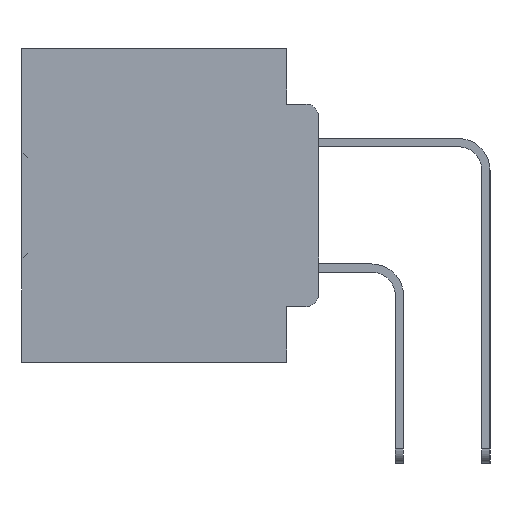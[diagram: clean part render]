
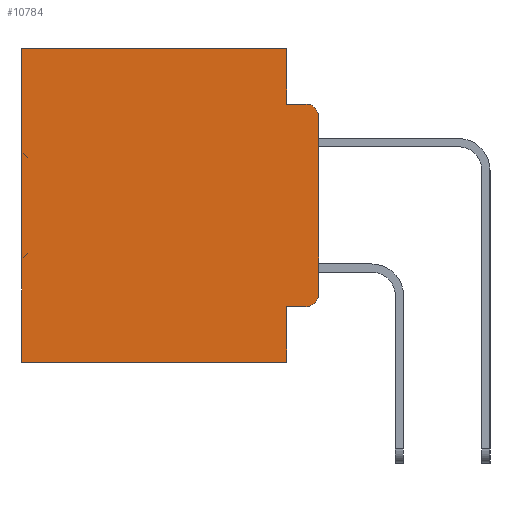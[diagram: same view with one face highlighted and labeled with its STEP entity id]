
A CAD part, left-side view. The second image highlights one B-rep face of the part: STEP entity #10784.
In plain terms, the highlighted planar face has unit normal (-1, 0, 0).
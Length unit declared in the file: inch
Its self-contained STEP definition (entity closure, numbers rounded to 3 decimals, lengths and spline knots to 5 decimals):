
#329 = DIRECTION ( 'NONE',  ( 0., 0., -1. ) ) ;
#488 = EDGE_LOOP ( 'NONE', ( #30533, #26511, #18700, #25436, #609, #20765, #15662, #32718, #24163, #22100 ) ) ;
#609 = ORIENTED_EDGE ( 'NONE', *, *, #13369, .T. ) ;
#620 = EDGE_CURVE ( 'NONE', #18896, #14443, #38742, .T. ) ;
#678 = CIRCLE ( 'NONE', #14601, 0.02 ) ;
#964 = CARTESIAN_POINT ( 'NONE',  ( 0.298, 0.473, 0. ) ) ;
#2478 = CIRCLE ( 'NONE', #34332, 0.02 ) ;
#3884 = VECTOR ( 'NONE', #29642, 39.37008 ) ;
#4218 = LINE ( 'NONE', #26890, #9497 ) ;
#4839 = CARTESIAN_POINT ( 'NONE',  ( 0.298, 0.473, -0.5 ) ) ;
#5211 = DIRECTION ( 'NONE',  ( 0., 0., -1. ) ) ;
#5315 = CARTESIAN_POINT ( 'NONE',  ( 0.298, 0.051, -0.5 ) ) ;
#6040 = CARTESIAN_POINT ( 'NONE',  ( 0.298, 0., -0.5 ) ) ;
#6179 = VERTEX_POINT ( 'NONE', #30960 ) ;
#8445 = CARTESIAN_POINT ( 'NONE',  ( 0.298, 0., 0. ) ) ;
#8889 = EDGE_CURVE ( 'NONE', #14443, #22047, #34363, .T. ) ;
#9144 = LINE ( 'NONE', #6040, #24581 ) ;
#9497 = VECTOR ( 'NONE', #23849, 39.37008 ) ;
#9655 = CARTESIAN_POINT ( 'NONE',  ( 0.298, 0.051, 0. ) ) ;
#9750 = DIRECTION ( 'NONE',  ( 0., 0., -1. ) ) ;
#10784 = ADVANCED_FACE ( 'NONE', ( #23888 ), #26889, .F. ) ;
#10981 = VERTEX_POINT ( 'NONE', #21712 ) ;
#10997 = EDGE_CURVE ( 'NONE', #10981, #22047, #678, .T. ) ;
#11593 = DIRECTION ( 'NONE',  ( 1., 0., 0. ) ) ;
#13076 = LINE ( 'NONE', #26604, #3884 ) ;
#13098 = VERTEX_POINT ( 'NONE', #28345 ) ;
#13369 = EDGE_CURVE ( 'NONE', #18896, #24915, #13076, .T. ) ;
#14443 = VERTEX_POINT ( 'NONE', #17045 ) ;
#14549 = VERTEX_POINT ( 'NONE', #29567 ) ;
#14601 = AXIS2_PLACEMENT_3D ( 'NONE', #37029, #18871, #329 ) ;
#15435 = CARTESIAN_POINT ( 'NONE',  ( 0.298, 0.473, 0. ) ) ;
#15662 = ORIENTED_EDGE ( 'NONE', *, *, #19798, .F. ) ;
#15744 = DIRECTION ( 'NONE',  ( -1., 0., 0. ) ) ;
#15890 = DIRECTION ( 'NONE',  ( 0., 0., -1. ) ) ;
#17045 = CARTESIAN_POINT ( 'NONE',  ( 0.298, 0.051, -0.0885 ) ) ;
#17214 = VECTOR ( 'NONE', #25278, 39.37008 ) ;
#17886 = VERTEX_POINT ( 'NONE', #4839 ) ;
#18629 = VECTOR ( 'NONE', #33732, 39.37008 ) ;
#18700 = ORIENTED_EDGE ( 'NONE', *, *, #8889, .F. ) ;
#18871 = DIRECTION ( 'NONE',  ( -1., 0., 0. ) ) ;
#18896 = VERTEX_POINT ( 'NONE', #35407 ) ;
#19022 = VECTOR ( 'NONE', #15890, 39.37008 ) ;
#19798 = EDGE_CURVE ( 'NONE', #36816, #17886, #9144, .T. ) ;
#20586 = CARTESIAN_POINT ( 'NONE',  ( 0.298, 0.051, 0. ) ) ;
#20765 = ORIENTED_EDGE ( 'NONE', *, *, #38309, .T. ) ;
#21433 = DIRECTION ( 'NONE',  ( 0., 1., 0. ) ) ;
#21712 = CARTESIAN_POINT ( 'NONE',  ( 0.298, 0., -0.1085 ) ) ;
#21994 = CARTESIAN_POINT ( 'NONE',  ( 0.298, 0., 0. ) ) ;
#22047 = VERTEX_POINT ( 'NONE', #27225 ) ;
#22100 = ORIENTED_EDGE ( 'NONE', *, *, #28215, .T. ) ;
#22395 = CARTESIAN_POINT ( 'NONE',  ( 0.298, 0.051, -0.0885 ) ) ;
#23403 = EDGE_CURVE ( 'NONE', #10981, #13098, #27128, .T. ) ;
#23849 = DIRECTION ( 'NONE',  ( 0., -1., 0. ) ) ;
#23888 = FACE_OUTER_BOUND ( 'NONE', #488, .T. ) ;
#24163 = ORIENTED_EDGE ( 'NONE', *, *, #30276, .T. ) ;
#24581 = VECTOR ( 'NONE', #21433, 39.37008 ) ;
#24915 = VERTEX_POINT ( 'NONE', #964 ) ;
#25278 = DIRECTION ( 'NONE',  ( 0., -1., 0. ) ) ;
#25436 = ORIENTED_EDGE ( 'NONE', *, *, #620, .F. ) ;
#25898 = VECTOR ( 'NONE', #5211, 39.37008 ) ;
#26511 = ORIENTED_EDGE ( 'NONE', *, *, #10997, .T. ) ;
#26604 = CARTESIAN_POINT ( 'NONE',  ( 0.298, 0., 0. ) ) ;
#26889 = PLANE ( 'NONE',  #29704 ) ;
#26890 = CARTESIAN_POINT ( 'NONE',  ( 0.298, 0.051, -0.4115 ) ) ;
#27128 = LINE ( 'NONE', #21994, #19022 ) ;
#27225 = CARTESIAN_POINT ( 'NONE',  ( 0.298, 0.02, -0.0885 ) ) ;
#28215 = EDGE_CURVE ( 'NONE', #14549, #13098, #2478, .T. ) ;
#28345 = CARTESIAN_POINT ( 'NONE',  ( 0.298, 0., -0.3915 ) ) ;
#29567 = CARTESIAN_POINT ( 'NONE',  ( 0.298, 0.02, -0.4115 ) ) ;
#29642 = DIRECTION ( 'NONE',  ( 0., 1., 0. ) ) ;
#29704 = AXIS2_PLACEMENT_3D ( 'NONE', #8445, #11593, #33002 ) ;
#30276 = EDGE_CURVE ( 'NONE', #6179, #14549, #4218, .T. ) ;
#30533 = ORIENTED_EDGE ( 'NONE', *, *, #23403, .F. ) ;
#30960 = CARTESIAN_POINT ( 'NONE',  ( 0.298, 0.051, -0.4115 ) ) ;
#32718 = ORIENTED_EDGE ( 'NONE', *, *, #36308, .F. ) ;
#33002 = DIRECTION ( 'NONE',  ( 0., 0., -1. ) ) ;
#33437 = VECTOR ( 'NONE', #9750, 39.37008 ) ;
#33732 = DIRECTION ( 'NONE',  ( 0., 0., -1. ) ) ;
#33860 = LINE ( 'NONE', #15435, #18629 ) ;
#34030 = CARTESIAN_POINT ( 'NONE',  ( 0.298, 0.02, -0.3915 ) ) ;
#34332 = AXIS2_PLACEMENT_3D ( 'NONE', #34030, #15744, #37031 ) ;
#34363 = LINE ( 'NONE', #22395, #17214 ) ;
#35407 = CARTESIAN_POINT ( 'NONE',  ( 0.298, 0.051, 0. ) ) ;
#35839 = LINE ( 'NONE', #20586, #25898 ) ;
#36308 = EDGE_CURVE ( 'NONE', #6179, #36816, #35839, .T. ) ;
#36816 = VERTEX_POINT ( 'NONE', #5315 ) ;
#37029 = CARTESIAN_POINT ( 'NONE',  ( 0.298, 0.02, -0.1085 ) ) ;
#37031 = DIRECTION ( 'NONE',  ( 0., 0., -1. ) ) ;
#38309 = EDGE_CURVE ( 'NONE', #24915, #17886, #33860, .T. ) ;
#38742 = LINE ( 'NONE', #9655, #33437 ) ;
